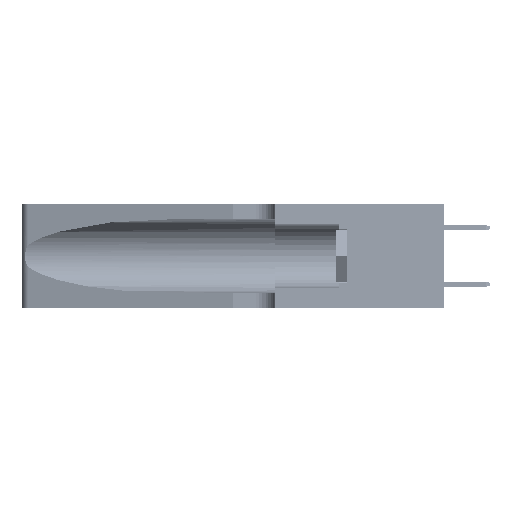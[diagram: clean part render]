
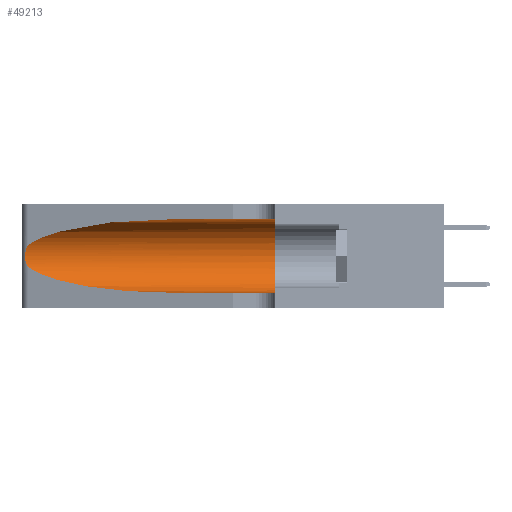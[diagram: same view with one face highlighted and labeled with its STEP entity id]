
A CAD part, left-side view. The second image highlights one B-rep face of the part: STEP entity #49213.
In plain terms, the highlighted cylindrical face has radius 3.308 mm (diameter 6.617 mm), a partial arc.
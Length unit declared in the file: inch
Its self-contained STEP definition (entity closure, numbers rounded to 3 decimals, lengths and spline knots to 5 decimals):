
#901 = EDGE_CURVE ( 'NONE', #4777, #38935, #38473, .T. ) ;
#1305 = ORIENTED_EDGE ( 'NONE', *, *, #45194, .T. ) ;
#1846 = CARTESIAN_POINT ( 'NONE',  ( 0.25487, 1.22718, 0.14631 ) ) ;
#2683 = CARTESIAN_POINT ( 'NONE',  ( 0.25639, 1.23184, 0.21858 ) ) ;
#4561 = CARTESIAN_POINT ( 'NONE',  ( 0.1305, 0.72297, 0.31525 ) ) ;
#4777 = VERTEX_POINT ( 'NONE', #12320 ) ;
#5213 = CARTESIAN_POINT ( 'NONE',  ( 0.1305, 0.35, 0.05475 ) ) ;
#5392 = CARTESIAN_POINT ( 'NONE',  ( 0.2373, 1.15595, 0.28018 ) ) ;
#5714 = DIRECTION ( 'NONE',  ( 0., 0., 1. ) ) ;
#6068 = DIRECTION ( 'NONE',  ( 0., 1., 0. ) ) ;
#6843 = CARTESIAN_POINT ( 'NONE',  ( 0.1305, 1.61858, 0.185 ) ) ;
#7183 = AXIS2_PLACEMENT_3D ( 'NONE', #6843, #27001, #47136 ) ;
#8613 = ORIENTED_EDGE ( 'NONE', *, *, #52272, .F. ) ;
#9092 =( BOUNDED_CURVE ( )  B_SPLINE_CURVE ( 3, ( #42299, #42478, #5392, #38378 ),
 .UNSPECIFIED., .F., .T. ) 
 B_SPLINE_CURVE_WITH_KNOTS ( ( 4, 4 ),
 ( 1.5708, 2.84003 ),
 .UNSPECIFIED. ) 
 CURVE ( )  GEOMETRIC_REPRESENTATION_ITEM ( )  RATIONAL_B_SPLINE_CURVE ( ( 1., 0.87, 0.87, 1. ) ) 
 REPRESENTATION_ITEM ( '' )  );
#9353 = LINE ( 'NONE', #46325, #25325 ) ;
#10353 = CARTESIAN_POINT ( 'NONE',  ( 0.1305, 0.35, 0.185 ) ) ;
#10591 = CARTESIAN_POINT ( 'NONE',  ( 0.1305, 0.72297, 0.05475 ) ) ;
#10814 = VECTOR ( 'NONE', #20749, 39.37008 ) ;
#11412 = CARTESIAN_POINT ( 'NONE',  ( 0.25789, 1.23486, 0.15765 ) ) ;
#11772 = CARTESIAN_POINT ( 'NONE',  ( 0.25555, 1.22993, 0.14849 ) ) ;
#12320 = CARTESIAN_POINT ( 'NONE',  ( 0.25487, 1.22718, 0.22369 ) ) ;
#13777 = EDGE_CURVE ( 'NONE', #14848, #41479, #47287, .T. ) ;
#14262 = CARTESIAN_POINT ( 'NONE',  ( 0.26018, 1.23835, 0.19895 ) ) ;
#14848 = VERTEX_POINT ( 'NONE', #25953 ) ;
#15300 = VERTEX_POINT ( 'NONE', #52479 ) ;
#15557 = FACE_OUTER_BOUND ( 'NONE', #41466, .T. ) ;
#15929 = LINE ( 'NONE', #32901, #10814 ) ;
#18531 = CARTESIAN_POINT ( 'NONE',  ( 0.25854, 1.2359, 0.20912 ) ) ;
#19617 = CARTESIAN_POINT ( 'NONE',  ( 0.25856, 1.23593, 0.16098 ) ) ;
#20749 = DIRECTION ( 'NONE',  ( 0., -1., 0. ) ) ;
#23381 = CARTESIAN_POINT ( 'NONE',  ( 0.25487, 1.22718, 0.14631 ) ) ;
#25325 = VECTOR ( 'NONE', #49528, 39.37008 ) ;
#25953 = CARTESIAN_POINT ( 'NONE',  ( 0.1305, 0.35, 0.31525 ) ) ;
#27001 = DIRECTION ( 'NONE',  ( 0., -1., 0. ) ) ;
#30695 = CARTESIAN_POINT ( 'NONE',  ( 0.26017, 1.23833, 0.17102 ) ) ;
#30727 = ORIENTED_EDGE ( 'NONE', *, *, #901, .T. ) ;
#31393 = CARTESIAN_POINT ( 'NONE',  ( 0.25555, 1.22994, 0.2215 ) ) ;
#31758 = CARTESIAN_POINT ( 'NONE',  ( 0.25639, 1.23186, 0.15144 ) ) ;
#32901 = CARTESIAN_POINT ( 'NONE',  ( 0.1305, 1.61858, 0.31525 ) ) ;
#34546 =( BOUNDED_CURVE ( )  B_SPLINE_CURVE ( 3, ( #47836, #51722, #39470, #10591 ),
 .UNSPECIFIED., .F., .F. ) 
 B_SPLINE_CURVE_WITH_KNOTS ( ( 4, 4 ),
 ( 3.44316, 4.71239 ),
 .UNSPECIFIED. ) 
 CURVE ( )  GEOMETRIC_REPRESENTATION_ITEM ( )  RATIONAL_B_SPLINE_CURVE ( ( 1., 0.87, 0.87, 1. ) ) 
 REPRESENTATION_ITEM ( '' )  );
#37643 = ORIENTED_EDGE ( 'NONE', *, *, #13777, .F. ) ;
#38378 = CARTESIAN_POINT ( 'NONE',  ( 0.25487, 1.22718, 0.22369 ) ) ;
#38473 = B_SPLINE_CURVE_WITH_KNOTS ( 'NONE', 3,
 ( #47611, #31393, #2683, #38709, #18531, #14262, #42813, #50951, #30695, #19617, #11412, #31758, #11772, #23381 ),
 .UNSPECIFIED., .F., .F.,
 ( 4, 2, 2, 2, 2, 2, 4 ),
 ( 0., 0.00027, 0.00053, 0.00107, 0.0016, 0.00187, 0.00214 ),
 .UNSPECIFIED. ) ;
#38709 = CARTESIAN_POINT ( 'NONE',  ( 0.25787, 1.23484, 0.2124 ) ) ;
#38752 = VERTEX_POINT ( 'NONE', #4561 ) ;
#38935 = VERTEX_POINT ( 'NONE', #1846 ) ;
#39470 = CARTESIAN_POINT ( 'NONE',  ( 0.18966, 0.96281, 0.05475 ) ) ;
#40214 = EDGE_CURVE ( 'NONE', #15300, #41479, #9353, .T. ) ;
#41435 = EDGE_CURVE ( 'NONE', #38752, #4777, #9092, .T. ) ;
#41466 = EDGE_LOOP ( 'NONE', ( #43559, #30727, #1305, #44155, #37643, #8613 ) ) ;
#41479 = VERTEX_POINT ( 'NONE', #5213 ) ;
#42299 = CARTESIAN_POINT ( 'NONE',  ( 0.1305, 0.72297, 0.31525 ) ) ;
#42478 = CARTESIAN_POINT ( 'NONE',  ( 0.18966, 0.96281, 0.31525 ) ) ;
#42813 = CARTESIAN_POINT ( 'NONE',  ( 0.26075, 1.23896, 0.19203 ) ) ;
#43559 = ORIENTED_EDGE ( 'NONE', *, *, #41435, .T. ) ;
#44155 = ORIENTED_EDGE ( 'NONE', *, *, #40214, .T. ) ;
#45194 = EDGE_CURVE ( 'NONE', #38935, #15300, #34546, .T. ) ;
#46325 = CARTESIAN_POINT ( 'NONE',  ( 0.1305, 1.61858, 0.05475 ) ) ;
#46814 = CYLINDRICAL_SURFACE ( 'NONE', #7183, 0.13025 ) ;
#47136 = DIRECTION ( 'NONE',  ( 0., 0., -1. ) ) ;
#47287 = CIRCLE ( 'NONE', #49488, 0.13025 ) ;
#47611 = CARTESIAN_POINT ( 'NONE',  ( 0.25487, 1.22718, 0.22369 ) ) ;
#47836 = CARTESIAN_POINT ( 'NONE',  ( 0.25487, 1.22718, 0.14631 ) ) ;
#49213 = ADVANCED_FACE ( 'NONE', ( #15557 ), #46814, .F. ) ;
#49488 = AXIS2_PLACEMENT_3D ( 'NONE', #10353, #6068, #5714 ) ;
#49528 = DIRECTION ( 'NONE',  ( 0., -1., 0. ) ) ;
#50951 = CARTESIAN_POINT ( 'NONE',  ( 0.26075, 1.23896, 0.178 ) ) ;
#51722 = CARTESIAN_POINT ( 'NONE',  ( 0.2373, 1.15595, 0.08982 ) ) ;
#52272 = EDGE_CURVE ( 'NONE', #38752, #14848, #15929, .T. ) ;
#52479 = CARTESIAN_POINT ( 'NONE',  ( 0.1305, 0.72297, 0.05475 ) ) ;
